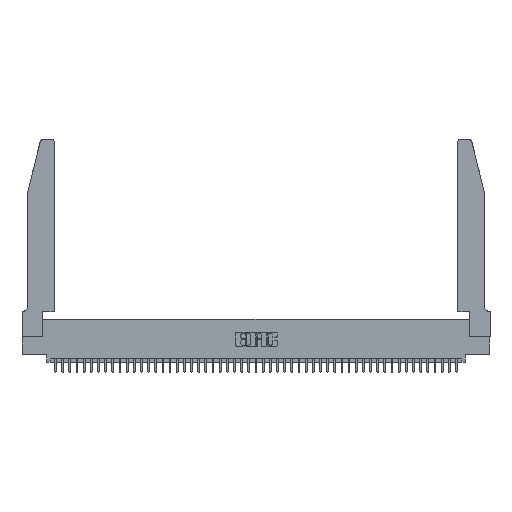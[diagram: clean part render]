
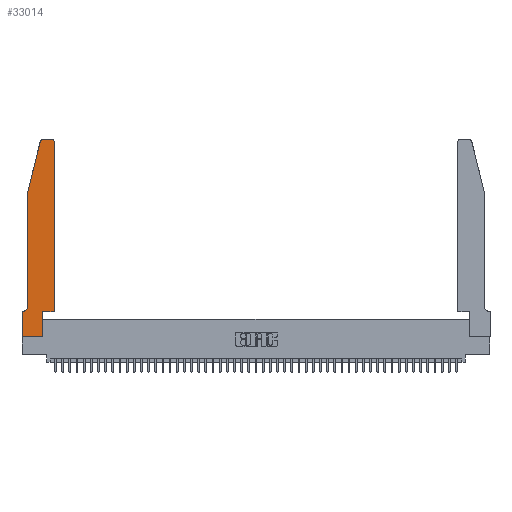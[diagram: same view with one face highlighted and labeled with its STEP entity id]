
A CAD part, top view. The second image highlights one B-rep face of the part: STEP entity #33014.
In plain terms, the highlighted planar face has unit normal (0, 0, 1).
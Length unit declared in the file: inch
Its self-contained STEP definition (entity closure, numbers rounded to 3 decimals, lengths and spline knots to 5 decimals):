
#328 = VERTEX_POINT ( 'NONE', #8418 ) ;
#1121 = ORIENTED_EDGE ( 'NONE', *, *, #39177, .T. ) ;
#1307 = DIRECTION ( 'NONE',  ( 1., 0., 0. ) ) ;
#2129 = CARTESIAN_POINT ( 'NONE',  ( 0.4505, 2.72, 0.37 ) ) ;
#2343 = CIRCLE ( 'NONE', #37521, 0.03 ) ;
#2437 = LINE ( 'NONE', #41043, #8700 ) ;
#2870 = EDGE_CURVE ( 'NONE', #4163, #14839, #41327, .T. ) ;
#4163 = VERTEX_POINT ( 'NONE', #30174 ) ;
#4342 = CARTESIAN_POINT ( 'NONE',  ( 0.0755, 2., 0.37 ) ) ;
#5271 = CARTESIAN_POINT ( 'NONE',  ( 0.2605, 2.75, 0.37 ) ) ;
#5852 = CARTESIAN_POINT ( 'NONE',  ( 0., 0., 0.37 ) ) ;
#7060 = VERTEX_POINT ( 'NONE', #36871 ) ;
#7697 = ORIENTED_EDGE ( 'NONE', *, *, #21900, .T. ) ;
#8026 = ORIENTED_EDGE ( 'NONE', *, *, #32455, .T. ) ;
#8345 = DIRECTION ( 'NONE',  ( -1., 0., 0. ) ) ;
#8418 = CARTESIAN_POINT ( 'NONE',  ( 0.25487, 2.72718, 0.37 ) ) ;
#8537 = ORIENTED_EDGE ( 'NONE', *, *, #11402, .T. ) ;
#8700 = VECTOR ( 'NONE', #34059, 39.37008 ) ;
#8741 = AXIS2_PLACEMENT_3D ( 'NONE', #19777, #27165, #1307 ) ;
#9255 = DIRECTION ( 'NONE',  ( -1., 0., 0. ) ) ;
#9552 = ORIENTED_EDGE ( 'NONE', *, *, #2870, .T. ) ;
#9701 = CARTESIAN_POINT ( 'NONE',  ( 0.0755, 0.42, 0.37 ) ) ;
#9903 = DIRECTION ( 'NONE',  ( 0., 0., 1. ) ) ;
#9946 = EDGE_CURVE ( 'NONE', #41261, #11199, #29544, .T. ) ;
#11199 = VERTEX_POINT ( 'NONE', #42080 ) ;
#11371 = CARTESIAN_POINT ( 'NONE',  ( 0.4205, 2.75, 0.37 ) ) ;
#11402 = EDGE_CURVE ( 'NONE', #18948, #18903, #20758, .T. ) ;
#12239 = EDGE_CURVE ( 'NONE', #11199, #328, #2343, .T. ) ;
#12890 = VECTOR ( 'NONE', #9255, 39.37008 ) ;
#12961 = CARTESIAN_POINT ( 'NONE',  ( 0.284, 2.72, 0.37 ) ) ;
#13951 = DIRECTION ( 'NONE',  ( 1., 0., 0. ) ) ;
#14525 = VECTOR ( 'NONE', #39449, 39.37008 ) ;
#14839 = VERTEX_POINT ( 'NONE', #2129 ) ;
#15026 = FACE_OUTER_BOUND ( 'NONE', #42931, .T. ) ;
#15377 = VERTEX_POINT ( 'NONE', #28566 ) ;
#17690 = DIRECTION ( 'NONE',  ( 0., 0., -1. ) ) ;
#18182 = VECTOR ( 'NONE', #18830, 39.37008 ) ;
#18830 = DIRECTION ( 'NONE',  ( -0.239, -0.971, 0. ) ) ;
#18903 = VERTEX_POINT ( 'NONE', #46091 ) ;
#18948 = VERTEX_POINT ( 'NONE', #41903 ) ;
#19777 = CARTESIAN_POINT ( 'NONE',  ( 0.4205, 2.72, 0.37 ) ) ;
#20189 = PLANE ( 'NONE',  #25827 ) ;
#20758 = LINE ( 'NONE', #47525, #21315 ) ;
#21315 = VECTOR ( 'NONE', #36702, 39.37008 ) ;
#21422 = ORIENTED_EDGE ( 'NONE', *, *, #45487, .T. ) ;
#21900 = EDGE_CURVE ( 'NONE', #328, #46550, #39554, .T. ) ;
#22898 = CARTESIAN_POINT ( 'NONE',  ( 0.0755, 0.35, 0.37 ) ) ;
#23443 = DIRECTION ( 'NONE',  ( 0., -1., 0. ) ) ;
#23613 = CARTESIAN_POINT ( 'NONE',  ( 0.0755, 2., 0.37 ) ) ;
#23970 = DIRECTION ( 'NONE',  ( 1., 0., 0. ) ) ;
#24204 = LINE ( 'NONE', #5852, #14525 ) ;
#24417 = ORIENTED_EDGE ( 'NONE', *, *, #34711, .T. ) ;
#25245 = CARTESIAN_POINT ( 'NONE',  ( 0.2865, 0.35, 0.37 ) ) ;
#25527 = ORIENTED_EDGE ( 'NONE', *, *, #9946, .T. ) ;
#25827 = AXIS2_PLACEMENT_3D ( 'NONE', #34687, #38419, #45999 ) ;
#25862 = VERTEX_POINT ( 'NONE', #9701 ) ;
#27165 = DIRECTION ( 'NONE',  ( 0., 0., 1. ) ) ;
#28566 = CARTESIAN_POINT ( 'NONE',  ( 0.0055, 0.35, 0.37 ) ) ;
#28791 = CARTESIAN_POINT ( 'NONE',  ( 0.0055, 0.42, 0.37 ) ) ;
#29139 = VERTEX_POINT ( 'NONE', #25245 ) ;
#29544 = LINE ( 'NONE', #5271, #12890 ) ;
#30174 = CARTESIAN_POINT ( 'NONE',  ( 0.4505, 0.35, 0.37 ) ) ;
#30990 = AXIS2_PLACEMENT_3D ( 'NONE', #28791, #17690, #43162 ) ;
#31330 = CIRCLE ( 'NONE', #8741, 0.03 ) ;
#32455 = EDGE_CURVE ( 'NONE', #18903, #7060, #24204, .T. ) ;
#33014 = ADVANCED_FACE ( 'NONE', ( #15026 ), #20189, .T. ) ;
#33319 = CARTESIAN_POINT ( 'NONE',  ( 0.0755, 2., 0.37 ) ) ;
#33427 = VECTOR ( 'NONE', #8345, 39.37008 ) ;
#33850 = VECTOR ( 'NONE', #23443, 39.37008 ) ;
#34059 = DIRECTION ( 'NONE',  ( 0., 1., 0. ) ) ;
#34687 = CARTESIAN_POINT ( 'NONE',  ( 0., 0.35, 0.37 ) ) ;
#34690 = EDGE_CURVE ( 'NONE', #7060, #29139, #2437, .T. ) ;
#34711 = EDGE_CURVE ( 'NONE', #15377, #18948, #35773, .T. ) ;
#34792 = CIRCLE ( 'NONE', #30990, 0.07 ) ;
#35033 = LINE ( 'NONE', #23613, #33850 ) ;
#35540 = VECTOR ( 'NONE', #39338, 39.37008 ) ;
#35773 = LINE ( 'NONE', #22898, #33427 ) ;
#36702 = DIRECTION ( 'NONE',  ( 0., -1., 0. ) ) ;
#36871 = CARTESIAN_POINT ( 'NONE',  ( 0.2865, 0., 0.37 ) ) ;
#37006 = EDGE_CURVE ( 'NONE', #46550, #25862, #35033, .T. ) ;
#37521 = AXIS2_PLACEMENT_3D ( 'NONE', #12961, #9903, #23970 ) ;
#38419 = DIRECTION ( 'NONE',  ( 0., 0., 1. ) ) ;
#39177 = EDGE_CURVE ( 'NONE', #14839, #41261, #31330, .T. ) ;
#39243 = ORIENTED_EDGE ( 'NONE', *, *, #34690, .T. ) ;
#39338 = DIRECTION ( 'NONE',  ( 0., 1., 0. ) ) ;
#39449 = DIRECTION ( 'NONE',  ( 1., 0., 0. ) ) ;
#39554 = LINE ( 'NONE', #33319, #18182 ) ;
#40005 = CARTESIAN_POINT ( 'NONE',  ( 0.4505, 0.35, 0.37 ) ) ;
#41043 = CARTESIAN_POINT ( 'NONE',  ( 0.2865, 0.35, 0.37 ) ) ;
#41261 = VERTEX_POINT ( 'NONE', #11371 ) ;
#41327 = LINE ( 'NONE', #42282, #35540 ) ;
#41798 = ORIENTED_EDGE ( 'NONE', *, *, #37006, .T. ) ;
#41903 = CARTESIAN_POINT ( 'NONE',  ( 0., 0.35, 0.37 ) ) ;
#42080 = CARTESIAN_POINT ( 'NONE',  ( 0.284, 2.75, 0.37 ) ) ;
#42282 = CARTESIAN_POINT ( 'NONE',  ( 0.4505, 0.35, 0.37 ) ) ;
#42374 = EDGE_CURVE ( 'NONE', #25862, #15377, #34792, .T. ) ;
#42931 = EDGE_LOOP ( 'NONE', ( #25527, #46183, #7697, #41798, #45756, #24417, #8537, #8026, #39243, #21422, #9552, #1121 ) ) ;
#43162 = DIRECTION ( 'NONE',  ( -1., 0., 0. ) ) ;
#43179 = VECTOR ( 'NONE', #13951, 39.37008 ) ;
#45487 = EDGE_CURVE ( 'NONE', #29139, #4163, #46607, .T. ) ;
#45756 = ORIENTED_EDGE ( 'NONE', *, *, #42374, .T. ) ;
#45999 = DIRECTION ( 'NONE',  ( 1., 0., 0. ) ) ;
#46091 = CARTESIAN_POINT ( 'NONE',  ( 0., 0., 0.37 ) ) ;
#46183 = ORIENTED_EDGE ( 'NONE', *, *, #12239, .T. ) ;
#46550 = VERTEX_POINT ( 'NONE', #4342 ) ;
#46607 = LINE ( 'NONE', #40005, #43179 ) ;
#47525 = CARTESIAN_POINT ( 'NONE',  ( 0., 0., 0.37 ) ) ;
